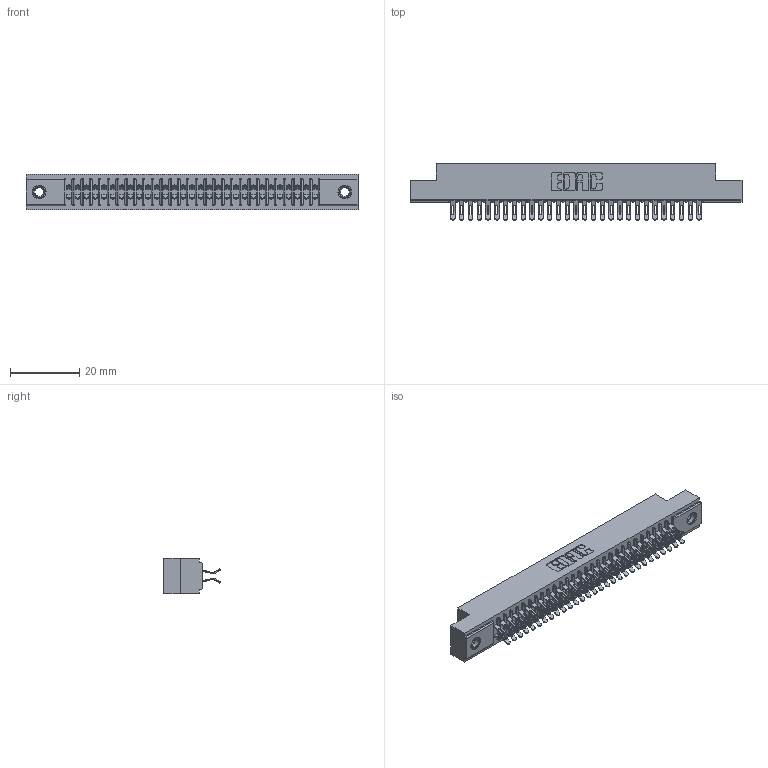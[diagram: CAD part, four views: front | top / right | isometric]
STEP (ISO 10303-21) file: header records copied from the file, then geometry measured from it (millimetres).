
FILE_DESCRIPTION (( 'STEP AP203' ), '1' );
FILE_NAME ('391-058-555-207.STEP', '2018-08-09T12:00:54', ( '' ), ( '' ), 'SwSTEP 2.0', 'SolidWorks 2016', '' );
FILE_SCHEMA (( 'CONFIG_CONTROL_DESIGN' ));
Length unit declared in the file: inch
Products named in the file (4): 391-058-555-207; 341 Part_.156 (3.96) Dia Mounting Holes; 341-292-001_341-292-155; 345-250-001_345-250-005-103
Assembly tree (61 placements, depth 2):
  391-058-555-207
    341 Part_.156 (3.96) Dia Mounting Holes
    341-292-001_341-292-155  x58
    345-250-001_345-250-005-103  x2
Bounding box: 95.89 x 16.31 x 10.16 mm (x, y, z)
Volume: 7129.3 mm3; surface area: 12753.7 mm2
Topology: 61 solids, 61 shells, 4700 faces, 13995 edges, 9106 vertices
Faces by surface type: plane 2536, cylinder 2032, sphere 60, torus 60, cone 12
Entity records: 38483 total; most frequent: CARTESIAN_POINT 6396, ORIENTED_EDGE 6338, DIRECTION 6217, EDGE_CURVE 3169, LINE 2527, VECTOR 2527, VERTEX_POINT 2008, AXIS2_PLACEMENT_3D 1845
